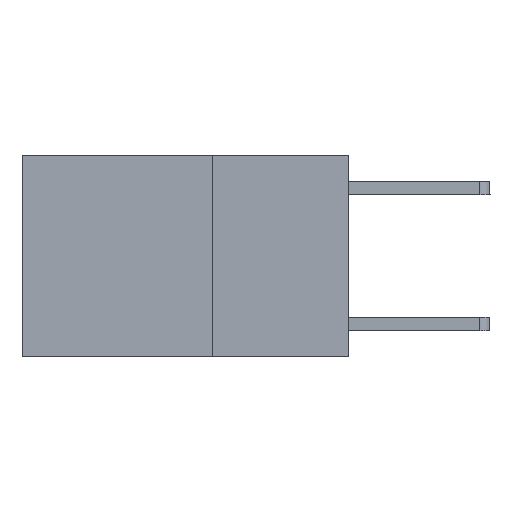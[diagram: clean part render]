
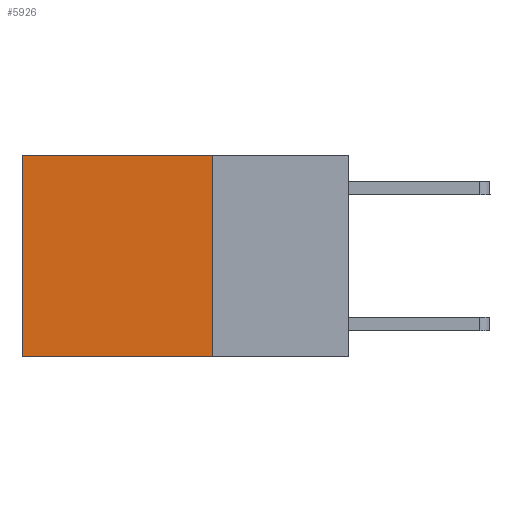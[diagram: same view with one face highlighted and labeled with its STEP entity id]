
A CAD part, left-side view. The second image highlights one B-rep face of the part: STEP entity #5926.
In plain terms, the highlighted planar face has unit normal (-1, 0, 0).
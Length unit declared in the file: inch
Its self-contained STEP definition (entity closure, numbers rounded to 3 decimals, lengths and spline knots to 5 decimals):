
#179 = LINE ( 'NONE', #4602, #11010 ) ;
#409 = DIRECTION ( 'NONE',  ( 0., 1., 0. ) ) ;
#835 = DIRECTION ( 'NONE',  ( 0., 0., -1. ) ) ;
#953 = EDGE_CURVE ( 'NONE', #6898, #10939, #7964, .T. ) ;
#1208 = DIRECTION ( 'NONE',  ( 0., 0., -1. ) ) ;
#1272 = AXIS2_PLACEMENT_3D ( 'NONE', #4844, #5791, #1208 ) ;
#1900 = ORIENTED_EDGE ( 'NONE', *, *, #8014, .F. ) ;
#2073 = LINE ( 'NONE', #2121, #7582 ) ;
#2083 = PLANE ( 'NONE',  #1272 ) ;
#2121 = CARTESIAN_POINT ( 'NONE',  ( 0.2625, 0.25, 0. ) ) ;
#2194 = FACE_OUTER_BOUND ( 'NONE', #3320, .T. ) ;
#3320 = EDGE_LOOP ( 'NONE', ( #5310, #6076, #1900, #9790 ) ) ;
#3574 = CARTESIAN_POINT ( 'NONE',  ( 0.2625, 0.25, 0. ) ) ;
#4602 = CARTESIAN_POINT ( 'NONE',  ( 0.2625, 0.6, 0. ) ) ;
#4630 = CARTESIAN_POINT ( 'NONE',  ( 0.2625, 0.6, -0.37 ) ) ;
#4631 = VERTEX_POINT ( 'NONE', #5423 ) ;
#4844 = CARTESIAN_POINT ( 'NONE',  ( 0.2625, 0.25, 0. ) ) ;
#4880 = VECTOR ( 'NONE', #5893, 39.37008 ) ;
#5310 = ORIENTED_EDGE ( 'NONE', *, *, #8727, .T. ) ;
#5423 = CARTESIAN_POINT ( 'NONE',  ( 0.2625, 0.6, 0. ) ) ;
#5791 = DIRECTION ( 'NONE',  ( 1., 0., 0. ) ) ;
#5893 = DIRECTION ( 'NONE',  ( 0., 1., 0. ) ) ;
#5926 = ADVANCED_FACE ( 'NONE', ( #2194 ), #2083, .F. ) ;
#5981 = VERTEX_POINT ( 'NONE', #6689 ) ;
#6076 = ORIENTED_EDGE ( 'NONE', *, *, #953, .F. ) ;
#6689 = CARTESIAN_POINT ( 'NONE',  ( 0.2625, 0.25, 0. ) ) ;
#6898 = VERTEX_POINT ( 'NONE', #8665 ) ;
#7582 = VECTOR ( 'NONE', #409, 39.37008 ) ;
#7964 = LINE ( 'NONE', #11482, #4880 ) ;
#8014 = EDGE_CURVE ( 'NONE', #5981, #6898, #11187, .T. ) ;
#8665 = CARTESIAN_POINT ( 'NONE',  ( 0.2625, 0.25, -0.37 ) ) ;
#8727 = EDGE_CURVE ( 'NONE', #4631, #10939, #179, .T. ) ;
#9267 = DIRECTION ( 'NONE',  ( 0., 0., -1. ) ) ;
#9632 = VECTOR ( 'NONE', #835, 39.37008 ) ;
#9790 = ORIENTED_EDGE ( 'NONE', *, *, #11920, .T. ) ;
#10939 = VERTEX_POINT ( 'NONE', #4630 ) ;
#11010 = VECTOR ( 'NONE', #9267, 39.37008 ) ;
#11187 = LINE ( 'NONE', #3574, #9632 ) ;
#11482 = CARTESIAN_POINT ( 'NONE',  ( 0.2625, 0.25, -0.37 ) ) ;
#11920 = EDGE_CURVE ( 'NONE', #5981, #4631, #2073, .T. ) ;
